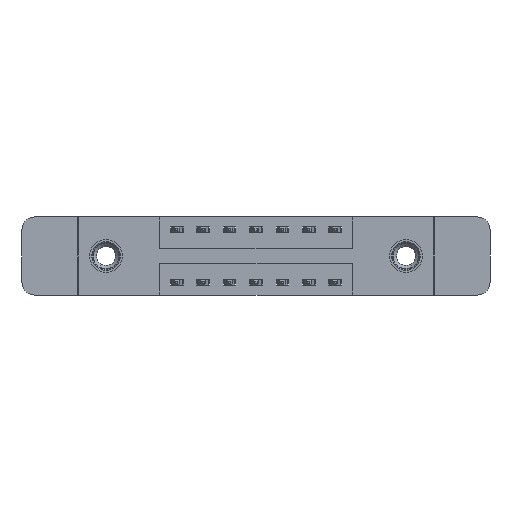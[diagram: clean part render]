
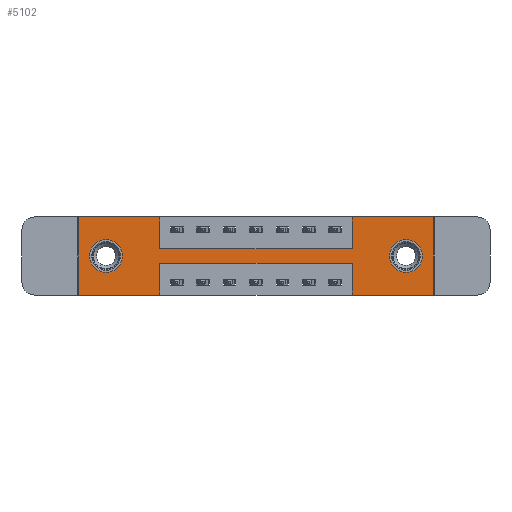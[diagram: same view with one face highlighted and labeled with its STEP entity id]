
A CAD part, front view. The second image highlights one B-rep face of the part: STEP entity #5102.
In plain terms, the highlighted planar face has unit normal (0, -1, 0).
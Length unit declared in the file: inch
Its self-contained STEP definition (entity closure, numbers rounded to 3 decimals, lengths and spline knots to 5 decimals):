
#89 = VERTEX_POINT ( 'NONE', #12019 ) ;
#102 = VECTOR ( 'NONE', #14082, 39.37008 ) ;
#272 = EDGE_LOOP ( 'NONE', ( #3315, #2188 ) ) ;
#397 = VECTOR ( 'NONE', #7658, 39.37008 ) ;
#406 = PLANE ( 'NONE',  #1872 ) ;
#497 = CARTESIAN_POINT ( 'NONE',  ( 1.2975, 0., -0.15 ) ) ;
#527 = CARTESIAN_POINT ( 'NONE',  ( 0.3875, 0., -0.37 ) ) ;
#663 = EDGE_CURVE ( 'NONE', #7581, #5040, #5451, .T. ) ;
#800 = CARTESIAN_POINT ( 'NONE',  ( 0., 0., 0. ) ) ;
#818 = VERTEX_POINT ( 'NONE', #4734 ) ;
#1272 = VERTEX_POINT ( 'NONE', #5618 ) ;
#1493 = VERTEX_POINT ( 'NONE', #11723 ) ;
#1698 = VECTOR ( 'NONE', #8660, 39.37008 ) ;
#1767 = LINE ( 'NONE', #527, #7690 ) ;
#1814 = LINE ( 'NONE', #4880, #5142 ) ;
#1872 = AXIS2_PLACEMENT_3D ( 'NONE', #12794, #13939, #11569 ) ;
#2025 = DIRECTION ( 'NONE',  ( 0., 0., -1. ) ) ;
#2171 = CARTESIAN_POINT ( 'NONE',  ( 1.5525, 0., -0.107 ) ) ;
#2188 = ORIENTED_EDGE ( 'NONE', *, *, #7274, .T. ) ;
#2601 = DIRECTION ( 'NONE',  ( 0., 1., 0. ) ) ;
#2670 = EDGE_CURVE ( 'NONE', #89, #1493, #3101, .T. ) ;
#2811 = DIRECTION ( 'NONE',  ( 0., 0., -1. ) ) ;
#2893 = CIRCLE ( 'NONE', #4967, 0.078 ) ;
#2937 = ORIENTED_EDGE ( 'NONE', *, *, #11573, .F. ) ;
#3069 = CARTESIAN_POINT ( 'NONE',  ( 1.685, 0., 0. ) ) ;
#3101 = LINE ( 'NONE', #12954, #102 ) ;
#3223 = CARTESIAN_POINT ( 'NONE',  ( 0., 0., -0.37 ) ) ;
#3315 = ORIENTED_EDGE ( 'NONE', *, *, #11544, .T. ) ;
#3587 = CARTESIAN_POINT ( 'NONE',  ( 0.1325, 0., -0.107 ) ) ;
#3811 = LINE ( 'NONE', #3069, #1698 ) ;
#3846 = CARTESIAN_POINT ( 'NONE',  ( 0.1325, 0., -0.185 ) ) ;
#3993 = VERTEX_POINT ( 'NONE', #5907 ) ;
#4002 = CARTESIAN_POINT ( 'NONE',  ( 0.3875, 0., -0.15 ) ) ;
#4005 = ORIENTED_EDGE ( 'NONE', *, *, #14231, .F. ) ;
#4058 = EDGE_CURVE ( 'NONE', #3993, #8356, #2893, .T. ) ;
#4103 = VERTEX_POINT ( 'NONE', #11779 ) ;
#4140 = VERTEX_POINT ( 'NONE', #800 ) ;
#4182 = CARTESIAN_POINT ( 'NONE',  ( 1.2975, 0., 0. ) ) ;
#4330 = ORIENTED_EDGE ( 'NONE', *, *, #5924, .F. ) ;
#4469 = DIRECTION ( 'NONE',  ( 0., 0., 1. ) ) ;
#4535 = CARTESIAN_POINT ( 'NONE',  ( 0.3875, 0., -0.15 ) ) ;
#4734 = CARTESIAN_POINT ( 'NONE',  ( 1.685, 0., -0.37 ) ) ;
#4814 = CARTESIAN_POINT ( 'NONE',  ( 1.2975, 0., -0.37 ) ) ;
#4880 = CARTESIAN_POINT ( 'NONE',  ( 1.2975, 0., -0.37 ) ) ;
#4967 = AXIS2_PLACEMENT_3D ( 'NONE', #4997, #7287, #5089 ) ;
#4984 = VECTOR ( 'NONE', #7129, 39.37008 ) ;
#4997 = CARTESIAN_POINT ( 'NONE',  ( 1.5525, 0., -0.185 ) ) ;
#5040 = VERTEX_POINT ( 'NONE', #497 ) ;
#5057 = EDGE_CURVE ( 'NONE', #7787, #4140, #8804, .T. ) ;
#5079 = EDGE_CURVE ( 'NONE', #7295, #89, #1814, .T. ) ;
#5089 = DIRECTION ( 'NONE',  ( 0., 0., -1. ) ) ;
#5102 = ADVANCED_FACE ( 'NONE', ( #7918, #6880, #13326 ), #406, .T. ) ;
#5142 = VECTOR ( 'NONE', #6072, 39.37008 ) ;
#5451 = LINE ( 'NONE', #4535, #11374 ) ;
#5558 = VECTOR ( 'NONE', #2025, 39.37008 ) ;
#5618 = CARTESIAN_POINT ( 'NONE',  ( 0.3875, 0., 0. ) ) ;
#5627 = ORIENTED_EDGE ( 'NONE', *, *, #13896, .T. ) ;
#5761 = ORIENTED_EDGE ( 'NONE', *, *, #9582, .F. ) ;
#5907 = CARTESIAN_POINT ( 'NONE',  ( 1.5525, 0., -0.263 ) ) ;
#5924 = EDGE_CURVE ( 'NONE', #7371, #7787, #13143, .T. ) ;
#6041 = CARTESIAN_POINT ( 'NONE',  ( 0., 0., 0. ) ) ;
#6072 = DIRECTION ( 'NONE',  ( 0., 0., 1. ) ) ;
#6148 = ORIENTED_EDGE ( 'NONE', *, *, #11985, .F. ) ;
#6305 = EDGE_LOOP ( 'NONE', ( #5627, #12339 ) ) ;
#6639 = EDGE_LOOP ( 'NONE', ( #10199, #11063, #7586, #6148, #12128, #2937, #12454, #13744, #4005, #5761, #11325, #4330 ) ) ;
#6684 = EDGE_CURVE ( 'NONE', #1493, #7371, #1767, .T. ) ;
#6746 = CARTESIAN_POINT ( 'NONE',  ( 0.1325, 0., -0.185 ) ) ;
#6795 = EDGE_CURVE ( 'NONE', #5040, #8685, #9472, .T. ) ;
#6880 = FACE_BOUND ( 'NONE', #272, .T. ) ;
#7129 = DIRECTION ( 'NONE',  ( 0., 0., 1. ) ) ;
#7240 = VERTEX_POINT ( 'NONE', #7706 ) ;
#7274 = EDGE_CURVE ( 'NONE', #4103, #9740, #12564, .T. ) ;
#7287 = DIRECTION ( 'NONE',  ( 0., 1., 0. ) ) ;
#7295 = VERTEX_POINT ( 'NONE', #4814 ) ;
#7371 = VERTEX_POINT ( 'NONE', #8042 ) ;
#7531 = CARTESIAN_POINT ( 'NONE',  ( 0., 0., -0.37 ) ) ;
#7581 = VERTEX_POINT ( 'NONE', #4002 ) ;
#7586 = ORIENTED_EDGE ( 'NONE', *, *, #5079, .F. ) ;
#7658 = DIRECTION ( 'NONE',  ( 1., 0., 0. ) ) ;
#7690 = VECTOR ( 'NONE', #2811, 39.37008 ) ;
#7706 = CARTESIAN_POINT ( 'NONE',  ( 1.685, 0., 0. ) ) ;
#7711 = CIRCLE ( 'NONE', #13722, 0.078 ) ;
#7787 = VERTEX_POINT ( 'NONE', #3223 ) ;
#7918 = FACE_BOUND ( 'NONE', #6305, .T. ) ;
#8042 = CARTESIAN_POINT ( 'NONE',  ( 0.3875, 0., -0.37 ) ) ;
#8356 = VERTEX_POINT ( 'NONE', #2171 ) ;
#8660 = DIRECTION ( 'NONE',  ( 0., 0., -1. ) ) ;
#8685 = VERTEX_POINT ( 'NONE', #4182 ) ;
#8765 = DIRECTION ( 'NONE',  ( 0., 0., 1. ) ) ;
#8804 = LINE ( 'NONE', #10613, #4984 ) ;
#8895 = DIRECTION ( 'NONE',  ( 0., 1., 0. ) ) ;
#9018 = CARTESIAN_POINT ( 'NONE',  ( 0., 0., -0.37 ) ) ;
#9233 = CIRCLE ( 'NONE', #9806, 0.078 ) ;
#9263 = DIRECTION ( 'NONE',  ( 0., 1., 0. ) ) ;
#9423 = DIRECTION ( 'NONE',  ( 1., 0., 0. ) ) ;
#9472 = LINE ( 'NONE', #14509, #12064 ) ;
#9582 = EDGE_CURVE ( 'NONE', #4140, #1272, #11251, .T. ) ;
#9740 = VERTEX_POINT ( 'NONE', #3587 ) ;
#9743 = CARTESIAN_POINT ( 'NONE',  ( 0.3875, 0., 0. ) ) ;
#9806 = AXIS2_PLACEMENT_3D ( 'NONE', #11568, #9263, #12694 ) ;
#10078 = DIRECTION ( 'NONE',  ( 1., 0., 0. ) ) ;
#10118 = DIRECTION ( 'NONE',  ( -1., 0., 0. ) ) ;
#10199 = ORIENTED_EDGE ( 'NONE', *, *, #6684, .F. ) ;
#10250 = LINE ( 'NONE', #9743, #5558 ) ;
#10430 = DIRECTION ( 'NONE',  ( 0., 0., 1. ) ) ;
#10613 = CARTESIAN_POINT ( 'NONE',  ( 0., 0., 0. ) ) ;
#10670 = AXIS2_PLACEMENT_3D ( 'NONE', #6746, #8895, #4469 ) ;
#10846 = LINE ( 'NONE', #9018, #13285 ) ;
#11063 = ORIENTED_EDGE ( 'NONE', *, *, #2670, .F. ) ;
#11251 = LINE ( 'NONE', #12155, #397 ) ;
#11325 = ORIENTED_EDGE ( 'NONE', *, *, #5057, .F. ) ;
#11374 = VECTOR ( 'NONE', #10078, 39.37008 ) ;
#11544 = EDGE_CURVE ( 'NONE', #9740, #4103, #7711, .T. ) ;
#11568 = CARTESIAN_POINT ( 'NONE',  ( 1.5525, 0., -0.185 ) ) ;
#11569 = DIRECTION ( 'NONE',  ( 0., 0., -1. ) ) ;
#11573 = EDGE_CURVE ( 'NONE', #8685, #7240, #13832, .T. ) ;
#11723 = CARTESIAN_POINT ( 'NONE',  ( 0.3875, 0., -0.22 ) ) ;
#11779 = CARTESIAN_POINT ( 'NONE',  ( 0.1325, 0., -0.263 ) ) ;
#11887 = VECTOR ( 'NONE', #9423, 39.37008 ) ;
#11985 = EDGE_CURVE ( 'NONE', #818, #7295, #10846, .T. ) ;
#12019 = CARTESIAN_POINT ( 'NONE',  ( 1.2975, 0., -0.22 ) ) ;
#12064 = VECTOR ( 'NONE', #8765, 39.37008 ) ;
#12083 = DIRECTION ( 'NONE',  ( -1., 0., 0. ) ) ;
#12128 = ORIENTED_EDGE ( 'NONE', *, *, #14240, .F. ) ;
#12155 = CARTESIAN_POINT ( 'NONE',  ( 0., 0., 0. ) ) ;
#12339 = ORIENTED_EDGE ( 'NONE', *, *, #4058, .T. ) ;
#12454 = ORIENTED_EDGE ( 'NONE', *, *, #6795, .F. ) ;
#12564 = CIRCLE ( 'NONE', #10670, 0.078 ) ;
#12694 = DIRECTION ( 'NONE',  ( 0., 0., -1. ) ) ;
#12794 = CARTESIAN_POINT ( 'NONE',  ( 0., 0., -0.37 ) ) ;
#12954 = CARTESIAN_POINT ( 'NONE',  ( 0.3875, 0., -0.22 ) ) ;
#13143 = LINE ( 'NONE', #7531, #13479 ) ;
#13285 = VECTOR ( 'NONE', #10118, 39.37008 ) ;
#13326 = FACE_OUTER_BOUND ( 'NONE', #6639, .T. ) ;
#13479 = VECTOR ( 'NONE', #12083, 39.37008 ) ;
#13722 = AXIS2_PLACEMENT_3D ( 'NONE', #3846, #2601, #10430 ) ;
#13744 = ORIENTED_EDGE ( 'NONE', *, *, #663, .F. ) ;
#13832 = LINE ( 'NONE', #6041, #11887 ) ;
#13896 = EDGE_CURVE ( 'NONE', #8356, #3993, #9233, .T. ) ;
#13939 = DIRECTION ( 'NONE',  ( 0., -1., 0. ) ) ;
#14082 = DIRECTION ( 'NONE',  ( -1., 0., 0. ) ) ;
#14231 = EDGE_CURVE ( 'NONE', #1272, #7581, #10250, .T. ) ;
#14240 = EDGE_CURVE ( 'NONE', #7240, #818, #3811, .T. ) ;
#14509 = CARTESIAN_POINT ( 'NONE',  ( 1.2975, 0., 0. ) ) ;
